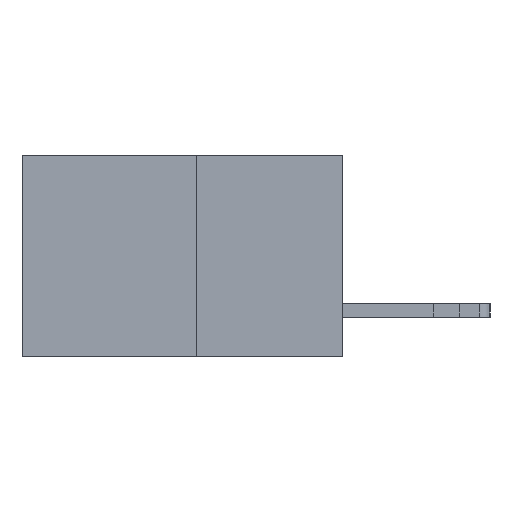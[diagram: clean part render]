
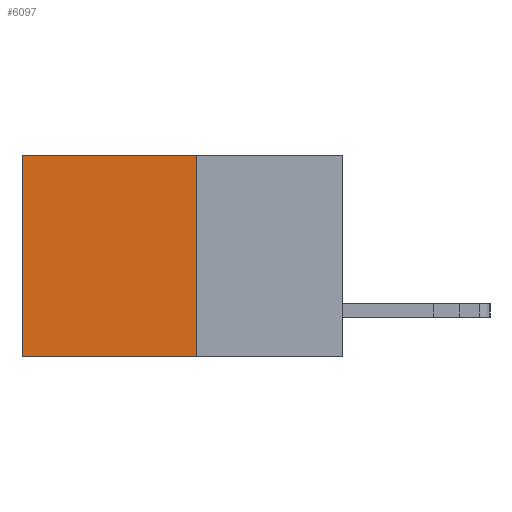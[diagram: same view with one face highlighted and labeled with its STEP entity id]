
A CAD part, left-side view. The second image highlights one B-rep face of the part: STEP entity #6097.
In plain terms, the highlighted planar face has unit normal (-1, 0, 0).
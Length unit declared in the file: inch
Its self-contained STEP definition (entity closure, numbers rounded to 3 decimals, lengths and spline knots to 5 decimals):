
#78 = AXIS2_PLACEMENT_3D ( 'NONE', #11151, #21622, #15778 ) ;
#178 = VECTOR ( 'NONE', #17167, 39.37008 ) ;
#467 = VERTEX_POINT ( 'NONE', #7272 ) ;
#1785 = CARTESIAN_POINT ( 'NONE',  ( 0.277, 0.59, -0.37 ) ) ;
#2393 = ORIENTED_EDGE ( 'NONE', *, *, #14000, .F. ) ;
#2570 = LINE ( 'NONE', #14212, #11109 ) ;
#2803 = CARTESIAN_POINT ( 'NONE',  ( 0.277, 0.59, 0. ) ) ;
#2921 = VERTEX_POINT ( 'NONE', #2803 ) ;
#4542 = VECTOR ( 'NONE', #12131, 39.37008 ) ;
#5219 = CARTESIAN_POINT ( 'NONE',  ( 0.277, 0.59, -0.37 ) ) ;
#5360 = VECTOR ( 'NONE', #7617, 39.37008 ) ;
#5885 = LINE ( 'NONE', #21864, #5360 ) ;
#6097 = ADVANCED_FACE ( 'NONE', ( #19290 ), #15808, .F. ) ;
#7160 = EDGE_CURVE ( 'NONE', #467, #2921, #5885, .T. ) ;
#7272 = CARTESIAN_POINT ( 'NONE',  ( 0.277, 0.27, 0. ) ) ;
#7617 = DIRECTION ( 'NONE',  ( 0., 1., 0. ) ) ;
#8454 = VERTEX_POINT ( 'NONE', #19162 ) ;
#8487 = LINE ( 'NONE', #5219, #4542 ) ;
#8999 = ORIENTED_EDGE ( 'NONE', *, *, #9717, .F. ) ;
#9274 = LINE ( 'NONE', #18776, #178 ) ;
#9717 = EDGE_CURVE ( 'NONE', #8454, #10858, #2570, .T. ) ;
#10858 = VERTEX_POINT ( 'NONE', #1785 ) ;
#11109 = VECTOR ( 'NONE', #20902, 39.37008 ) ;
#11151 = CARTESIAN_POINT ( 'NONE',  ( 0.277, 0.27, -0.37 ) ) ;
#12131 = DIRECTION ( 'NONE',  ( 0., 0., -1. ) ) ;
#12901 = ORIENTED_EDGE ( 'NONE', *, *, #7160, .T. ) ;
#13384 = EDGE_CURVE ( 'NONE', #2921, #10858, #8487, .T. ) ;
#14000 = EDGE_CURVE ( 'NONE', #467, #8454, #9274, .T. ) ;
#14212 = CARTESIAN_POINT ( 'NONE',  ( 0.277, 0.27, -0.37 ) ) ;
#15553 = EDGE_LOOP ( 'NONE', ( #22122, #8999, #2393, #12901 ) ) ;
#15778 = DIRECTION ( 'NONE',  ( 0., 0., -1. ) ) ;
#15808 = PLANE ( 'NONE',  #78 ) ;
#17167 = DIRECTION ( 'NONE',  ( 0., 0., -1. ) ) ;
#18776 = CARTESIAN_POINT ( 'NONE',  ( 0.277, 0.27, -0.37 ) ) ;
#19162 = CARTESIAN_POINT ( 'NONE',  ( 0.277, 0.27, -0.37 ) ) ;
#19290 = FACE_OUTER_BOUND ( 'NONE', #15553, .T. ) ;
#20902 = DIRECTION ( 'NONE',  ( 0., 1., 0. ) ) ;
#21622 = DIRECTION ( 'NONE',  ( 1., 0., 0. ) ) ;
#21864 = CARTESIAN_POINT ( 'NONE',  ( 0.277, 0.27, 0. ) ) ;
#22122 = ORIENTED_EDGE ( 'NONE', *, *, #13384, .T. ) ;
